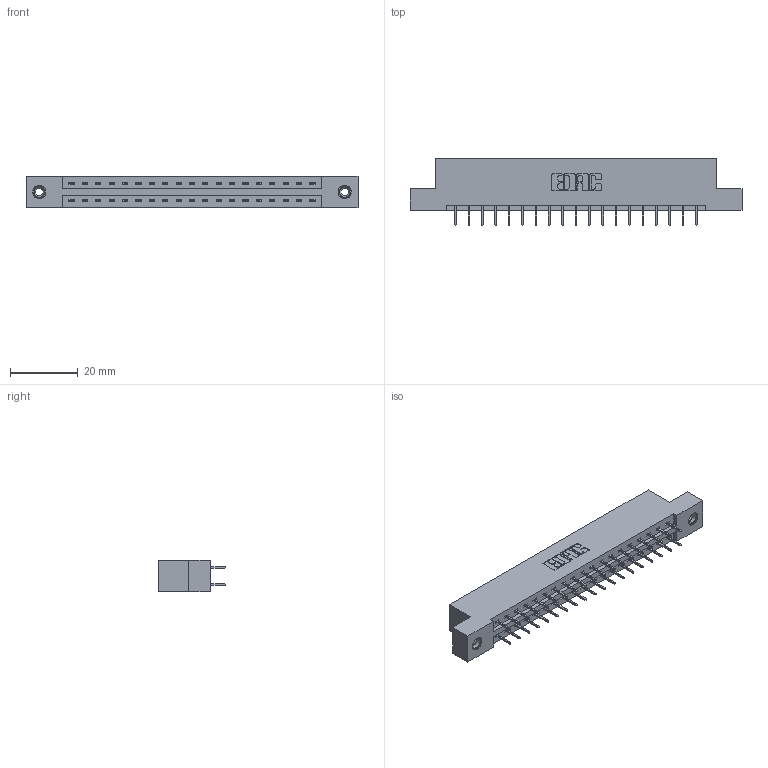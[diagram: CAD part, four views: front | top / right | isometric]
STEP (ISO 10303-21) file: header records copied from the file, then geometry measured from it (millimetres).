
FILE_DESCRIPTION (( 'STEP AP203' ), '1' );
FILE_NAME ('387-038-524-208.STEP', '2019-10-17T21:10:26', ( '' ), ( '' ), 'SwSTEP 2.0', 'SolidWorks 2016', '' );
FILE_SCHEMA (( 'CONFIG_CONTROL_DESIGN' ));
Length unit declared in the file: inch
Products named in the file (4): 337 Part_Flush Mounting Lugs - 0.156 Dia-TI; 345-250-001_345-250-003-102; 387-038-524-208; 345-292-001_345-293-124
Assembly tree (41 placements, depth 2):
  387-038-524-208
    337 Part_Flush Mounting Lugs - 0.156 Dia-TI
    345-292-001_345-293-124  x38
    345-250-001_345-250-003-102  x2
Bounding box: 98.3 x 19.69 x 9.4 mm (x, y, z)
Volume: 9989.2 mm3; surface area: 10915.3 mm2
Topology: 41 solids, 41 shells, 2378 faces, 6717 edges, 4318 vertices
Faces by surface type: plane 1774, cylinder 588, cone 12, torus 4
Entity records: 18966 total; most frequent: CARTESIAN_POINT 3193, ORIENTED_EDGE 3122, DIRECTION 2791, EDGE_CURVE 1561, LINE 1417, VECTOR 1417, VERTEX_POINT 1032, AXIS2_PLACEMENT_3D 687
